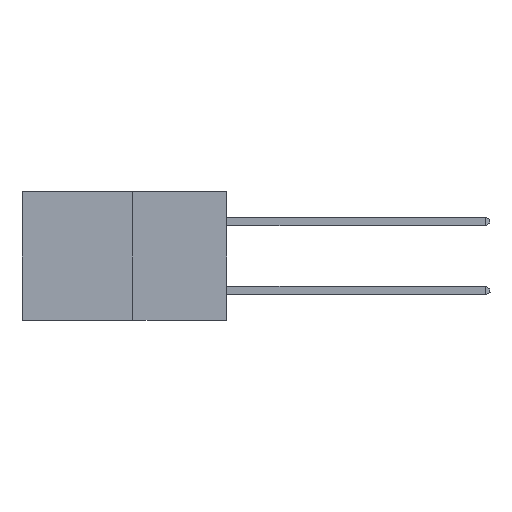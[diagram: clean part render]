
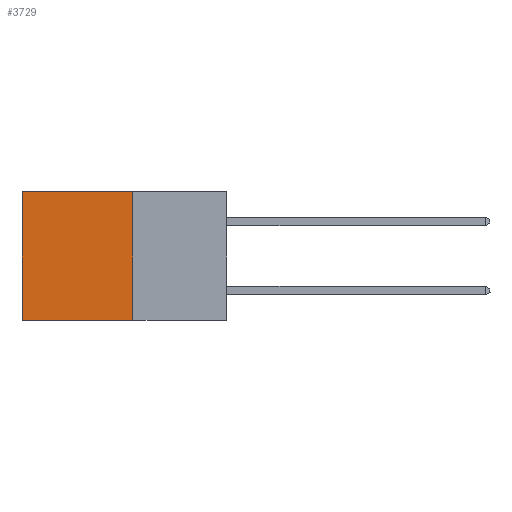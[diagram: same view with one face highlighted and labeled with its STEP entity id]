
A CAD part, left-side view. The second image highlights one B-rep face of the part: STEP entity #3729.
In plain terms, the highlighted planar face has unit normal (-1, 0, 0).
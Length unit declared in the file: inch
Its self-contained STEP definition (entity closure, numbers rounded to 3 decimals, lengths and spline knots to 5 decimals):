
#2101 = EDGE_CURVE ( 'NONE', #27485, #16287, #23047, .T. ) ;
#2242 = VECTOR ( 'NONE', #17524, 39.37008 ) ;
#3052 = DIRECTION ( 'NONE',  ( 0., 0., -1. ) ) ;
#3729 = ADVANCED_FACE ( 'NONE', ( #22545 ), #13357, .F. ) ;
#5635 = LINE ( 'NONE', #21088, #32259 ) ;
#6270 = LINE ( 'NONE', #8016, #19273 ) ;
#8010 = EDGE_LOOP ( 'NONE', ( #9212, #25885, #18351, #14960 ) ) ;
#8016 = CARTESIAN_POINT ( 'NONE',  ( 0.277, 0.27, -0.37 ) ) ;
#8949 = EDGE_CURVE ( 'NONE', #20350, #27485, #31761, .T. ) ;
#9212 = ORIENTED_EDGE ( 'NONE', *, *, #2101, .T. ) ;
#10667 = DIRECTION ( 'NONE',  ( 0., 1., 0. ) ) ;
#11380 = VERTEX_POINT ( 'NONE', #22446 ) ;
#13357 = PLANE ( 'NONE',  #31170 ) ;
#13748 = CARTESIAN_POINT ( 'NONE',  ( 0.277, 0.59, 0. ) ) ;
#14960 = ORIENTED_EDGE ( 'NONE', *, *, #8949, .T. ) ;
#16287 = VERTEX_POINT ( 'NONE', #19836 ) ;
#17524 = DIRECTION ( 'NONE',  ( 0., 0., -1. ) ) ;
#18351 = ORIENTED_EDGE ( 'NONE', *, *, #26272, .F. ) ;
#19273 = VECTOR ( 'NONE', #10667, 39.37008 ) ;
#19836 = CARTESIAN_POINT ( 'NONE',  ( 0.277, 0.59, -0.37 ) ) ;
#20045 = CARTESIAN_POINT ( 'NONE',  ( 0.277, 0.27, 0. ) ) ;
#20350 = VERTEX_POINT ( 'NONE', #20045 ) ;
#21088 = CARTESIAN_POINT ( 'NONE',  ( 0.277, 0.27, -0.37 ) ) ;
#22446 = CARTESIAN_POINT ( 'NONE',  ( 0.277, 0.27, -0.37 ) ) ;
#22545 = FACE_OUTER_BOUND ( 'NONE', #8010, .T. ) ;
#23047 = LINE ( 'NONE', #28200, #2242 ) ;
#23321 = DIRECTION ( 'NONE',  ( 0., 0., -1. ) ) ;
#24263 = VECTOR ( 'NONE', #30260, 39.37008 ) ;
#25722 = CARTESIAN_POINT ( 'NONE',  ( 0.277, 0.27, -0.37 ) ) ;
#25885 = ORIENTED_EDGE ( 'NONE', *, *, #31476, .F. ) ;
#26272 = EDGE_CURVE ( 'NONE', #20350, #11380, #5635, .T. ) ;
#27485 = VERTEX_POINT ( 'NONE', #13748 ) ;
#28200 = CARTESIAN_POINT ( 'NONE',  ( 0.277, 0.59, -0.37 ) ) ;
#30260 = DIRECTION ( 'NONE',  ( 0., 1., 0. ) ) ;
#31084 = DIRECTION ( 'NONE',  ( 1., 0., 0. ) ) ;
#31170 = AXIS2_PLACEMENT_3D ( 'NONE', #25722, #31084, #23321 ) ;
#31476 = EDGE_CURVE ( 'NONE', #11380, #16287, #6270, .T. ) ;
#31761 = LINE ( 'NONE', #32661, #24263 ) ;
#32259 = VECTOR ( 'NONE', #3052, 39.37008 ) ;
#32661 = CARTESIAN_POINT ( 'NONE',  ( 0.277, 0.27, 0. ) ) ;
